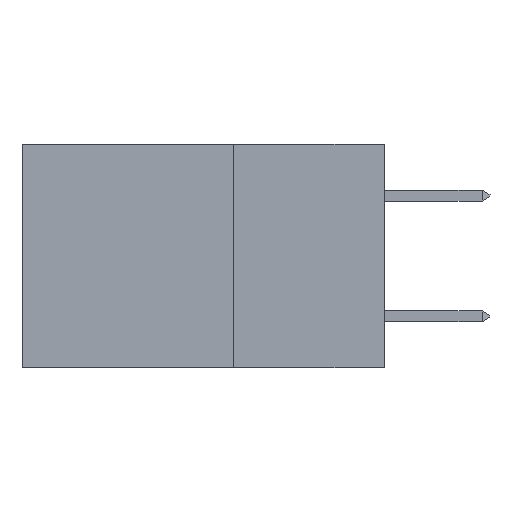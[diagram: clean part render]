
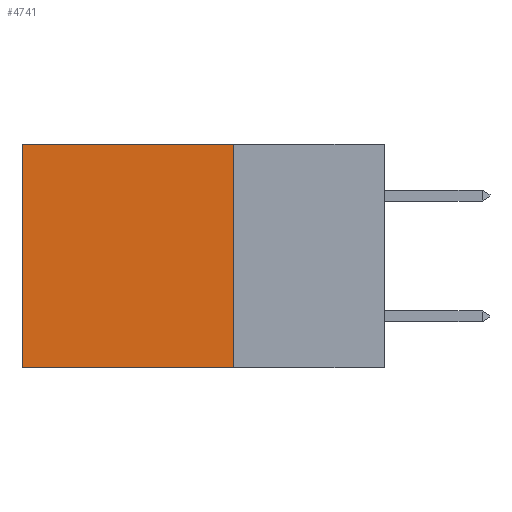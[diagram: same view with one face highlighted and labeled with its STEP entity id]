
A CAD part, left-side view. The second image highlights one B-rep face of the part: STEP entity #4741.
In plain terms, the highlighted planar face has unit normal (-1, 0, 0).
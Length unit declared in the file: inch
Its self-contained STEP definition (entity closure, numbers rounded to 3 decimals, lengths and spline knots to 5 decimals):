
#35 = CARTESIAN_POINT ( 'NONE',  ( 0.2875, 0.25, 0. ) ) ;
#357 = LINE ( 'NONE', #35, #8373 ) ;
#365 = DIRECTION ( 'NONE',  ( 0., 0., -1. ) ) ;
#747 = ORIENTED_EDGE ( 'NONE', *, *, #1223, .T. ) ;
#866 = VECTOR ( 'NONE', #7179, 39.37008 ) ;
#1223 = EDGE_CURVE ( 'NONE', #5541, #3152, #9056, .T. ) ;
#1602 = VERTEX_POINT ( 'NONE', #10109 ) ;
#1774 = ORIENTED_EDGE ( 'NONE', *, *, #9318, .T. ) ;
#2676 = LINE ( 'NONE', #6542, #2963 ) ;
#2963 = VECTOR ( 'NONE', #7259, 39.37008 ) ;
#3152 = VERTEX_POINT ( 'NONE', #9007 ) ;
#3300 = CARTESIAN_POINT ( 'NONE',  ( 0.2875, 0.25, 0. ) ) ;
#3349 = VECTOR ( 'NONE', #8328, 39.37008 ) ;
#3410 = ORIENTED_EDGE ( 'NONE', *, *, #6355, .F. ) ;
#4741 = ADVANCED_FACE ( 'NONE', ( #8175 ), #4942, .F. ) ;
#4942 = PLANE ( 'NONE',  #5333 ) ;
#5281 = VERTEX_POINT ( 'NONE', #10236 ) ;
#5333 = AXIS2_PLACEMENT_3D ( 'NONE', #3300, #5741, #365 ) ;
#5541 = VERTEX_POINT ( 'NONE', #9796 ) ;
#5741 = DIRECTION ( 'NONE',  ( 1., 0., 0. ) ) ;
#5812 = LINE ( 'NONE', #6450, #866 ) ;
#6355 = EDGE_CURVE ( 'NONE', #5281, #3152, #2676, .T. ) ;
#6450 = CARTESIAN_POINT ( 'NONE',  ( 0.2875, 0.25, 0. ) ) ;
#6542 = CARTESIAN_POINT ( 'NONE',  ( 0.2875, 0.25, -0.37 ) ) ;
#6907 = ORIENTED_EDGE ( 'NONE', *, *, #9057, .F. ) ;
#7179 = DIRECTION ( 'NONE',  ( 0., 1., 0. ) ) ;
#7259 = DIRECTION ( 'NONE',  ( 0., 1., 0. ) ) ;
#7710 = DIRECTION ( 'NONE',  ( 0., 0., -1. ) ) ;
#7776 = EDGE_LOOP ( 'NONE', ( #747, #3410, #6907, #1774 ) ) ;
#8175 = FACE_OUTER_BOUND ( 'NONE', #7776, .T. ) ;
#8328 = DIRECTION ( 'NONE',  ( 0., 0., -1. ) ) ;
#8373 = VECTOR ( 'NONE', #7710, 39.37008 ) ;
#8715 = CARTESIAN_POINT ( 'NONE',  ( 0.2875, 0.6, 0. ) ) ;
#9007 = CARTESIAN_POINT ( 'NONE',  ( 0.2875, 0.6, -0.37 ) ) ;
#9056 = LINE ( 'NONE', #8715, #3349 ) ;
#9057 = EDGE_CURVE ( 'NONE', #1602, #5281, #357, .T. ) ;
#9318 = EDGE_CURVE ( 'NONE', #1602, #5541, #5812, .T. ) ;
#9796 = CARTESIAN_POINT ( 'NONE',  ( 0.2875, 0.6, 0. ) ) ;
#10109 = CARTESIAN_POINT ( 'NONE',  ( 0.2875, 0.25, 0. ) ) ;
#10236 = CARTESIAN_POINT ( 'NONE',  ( 0.2875, 0.25, -0.37 ) ) ;
